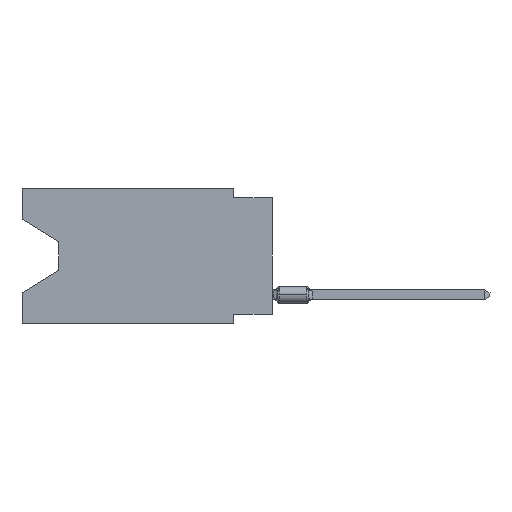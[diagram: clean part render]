
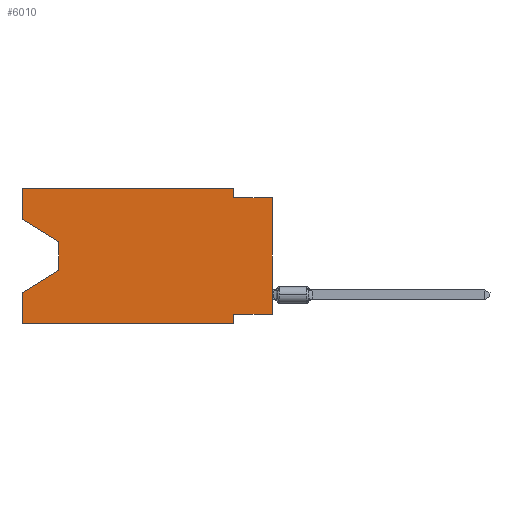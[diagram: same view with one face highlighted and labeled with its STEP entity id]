
A CAD part, left-side view. The second image highlights one B-rep face of the part: STEP entity #6010.
In plain terms, the highlighted planar face has unit normal (-1, 0, 0).
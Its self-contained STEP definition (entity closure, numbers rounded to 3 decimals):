
#204 = VERTEX_POINT ( 'NONE', #6367 ) ;
#647 = DIRECTION ( 'NONE',  ( 0., 1., 0. ) ) ;
#783 = CARTESIAN_POINT ( 'NONE',  ( 0., 0., 0. ) ) ;
#834 = LINE ( 'NONE', #11885, #6127 ) ;
#992 = VECTOR ( 'NONE', #4723, 1000. ) ;
#1112 = ORIENTED_EDGE ( 'NONE', *, *, #3923, .T. ) ;
#1198 = DIRECTION ( 'NONE',  ( 0., 0.855, -0.519 ) ) ;
#1315 = LINE ( 'NONE', #16510, #1983 ) ;
#1483 = CARTESIAN_POINT ( 'NONE',  ( 0., 16.383, -8.89 ) ) ;
#1664 = VECTOR ( 'NONE', #13502, 1000. ) ;
#1983 = VECTOR ( 'NONE', #8372, 1000. ) ;
#2185 = ORIENTED_EDGE ( 'NONE', *, *, #11172, .F. ) ;
#2428 = EDGE_CURVE ( 'NONE', #12531, #3201, #16859, .T. ) ;
#2451 = LINE ( 'NONE', #14931, #11621 ) ;
#2608 = ORIENTED_EDGE ( 'NONE', *, *, #7534, .F. ) ;
#3176 = VERTEX_POINT ( 'NONE', #9819 ) ;
#3201 = VERTEX_POINT ( 'NONE', #9553 ) ;
#3488 = EDGE_CURVE ( 'NONE', #3720, #14097, #834, .T. ) ;
#3533 = ORIENTED_EDGE ( 'NONE', *, *, #11182, .F. ) ;
#3636 = DIRECTION ( 'NONE',  ( 0., 0., 1. ) ) ;
#3705 = CARTESIAN_POINT ( 'NONE',  ( 0., 2.54, -8.89 ) ) ;
#3720 = VERTEX_POINT ( 'NONE', #14129 ) ;
#3766 = FACE_OUTER_BOUND ( 'NONE', #9793, .T. ) ;
#3818 = CARTESIAN_POINT ( 'NONE',  ( 0., 16.383, 0. ) ) ;
#3923 = EDGE_CURVE ( 'NONE', #12180, #12531, #2451, .T. ) ;
#4723 = DIRECTION ( 'NONE',  ( 0., 0., -1. ) ) ;
#4765 = DIRECTION ( 'NONE',  ( 0., 0., 1. ) ) ;
#4813 = VERTEX_POINT ( 'NONE', #16566 ) ;
#5173 = CARTESIAN_POINT ( 'NONE',  ( 0., 16.383, 0. ) ) ;
#5475 = DIRECTION ( 'NONE',  ( 1., 0., 0. ) ) ;
#5490 = CARTESIAN_POINT ( 'NONE',  ( 0., 2.54, 0. ) ) ;
#6010 = ADVANCED_FACE ( 'NONE', ( #3766 ), #17866, .F. ) ;
#6127 = VECTOR ( 'NONE', #647, 1000. ) ;
#6319 = LINE ( 'NONE', #783, #9073 ) ;
#6367 = CARTESIAN_POINT ( 'NONE',  ( 0., 16.383, -6.852 ) ) ;
#6377 = VERTEX_POINT ( 'NONE', #9716 ) ;
#6419 = LINE ( 'NONE', #13300, #14679 ) ;
#6822 = ORIENTED_EDGE ( 'NONE', *, *, #3488, .F. ) ;
#6824 = CARTESIAN_POINT ( 'NONE',  ( 0., 13.97, -5.385 ) ) ;
#6936 = DIRECTION ( 'NONE',  ( 0., 0., -1. ) ) ;
#7210 = CARTESIAN_POINT ( 'NONE',  ( 0., 2.54, -8.255 ) ) ;
#7383 = VERTEX_POINT ( 'NONE', #14224 ) ;
#7534 = EDGE_CURVE ( 'NONE', #12180, #4813, #7885, .T. ) ;
#7779 = DIRECTION ( 'NONE',  ( 0., 0., -1. ) ) ;
#7885 = LINE ( 'NONE', #5173, #16621 ) ;
#8364 = EDGE_CURVE ( 'NONE', #3201, #204, #9628, .T. ) ;
#8372 = DIRECTION ( 'NONE',  ( 0., 0., 1. ) ) ;
#8445 = AXIS2_PLACEMENT_3D ( 'NONE', #16250, #5475, #17686 ) ;
#8815 = CARTESIAN_POINT ( 'NONE',  ( 0., 13.97, -3.505 ) ) ;
#8919 = VECTOR ( 'NONE', #1198, 1000. ) ;
#9073 = VECTOR ( 'NONE', #4765, 1000. ) ;
#9150 = CARTESIAN_POINT ( 'NONE',  ( 0., 0., -0.635 ) ) ;
#9553 = CARTESIAN_POINT ( 'NONE',  ( 0., 13.97, -5.385 ) ) ;
#9628 = LINE ( 'NONE', #6824, #8919 ) ;
#9716 = CARTESIAN_POINT ( 'NONE',  ( 0., 2.54, -0.635 ) ) ;
#9793 = EDGE_LOOP ( 'NONE', ( #1112, #13552, #10392, #10011, #17423, #3533, #6822, #10310, #2185, #11666, #12014, #2608 ) ) ;
#9819 = CARTESIAN_POINT ( 'NONE',  ( 0., 2.54, 0. ) ) ;
#10011 = ORIENTED_EDGE ( 'NONE', *, *, #14334, .F. ) ;
#10019 = VERTEX_POINT ( 'NONE', #9150 ) ;
#10310 = ORIENTED_EDGE ( 'NONE', *, *, #15839, .T. ) ;
#10392 = ORIENTED_EDGE ( 'NONE', *, *, #8364, .T. ) ;
#10852 = VECTOR ( 'NONE', #6936, 1000. ) ;
#10859 = DIRECTION ( 'NONE',  ( 0., -1., 0. ) ) ;
#11172 = EDGE_CURVE ( 'NONE', #6377, #10019, #6419, .T. ) ;
#11182 = EDGE_CURVE ( 'NONE', #14097, #13721, #16277, .T. ) ;
#11621 = VECTOR ( 'NONE', #13398, 1000. ) ;
#11666 = ORIENTED_EDGE ( 'NONE', *, *, #16131, .F. ) ;
#11885 = CARTESIAN_POINT ( 'NONE',  ( 0., 0., -8.255 ) ) ;
#12014 = ORIENTED_EDGE ( 'NONE', *, *, #12551, .F. ) ;
#12160 = CARTESIAN_POINT ( 'NONE',  ( 0., 2.54, -8.89 ) ) ;
#12180 = VERTEX_POINT ( 'NONE', #16938 ) ;
#12291 = LINE ( 'NONE', #5490, #10852 ) ;
#12531 = VERTEX_POINT ( 'NONE', #16300 ) ;
#12551 = EDGE_CURVE ( 'NONE', #4813, #3176, #15033, .T. ) ;
#13300 = CARTESIAN_POINT ( 'NONE',  ( 0., 0., -0.635 ) ) ;
#13398 = DIRECTION ( 'NONE',  ( 0., -0.855, -0.519 ) ) ;
#13502 = DIRECTION ( 'NONE',  ( 0., -1., 0. ) ) ;
#13552 = ORIENTED_EDGE ( 'NONE', *, *, #2428, .T. ) ;
#13721 = VERTEX_POINT ( 'NONE', #12160 ) ;
#14097 = VERTEX_POINT ( 'NONE', #7210 ) ;
#14129 = CARTESIAN_POINT ( 'NONE',  ( 0., 0., -8.255 ) ) ;
#14224 = CARTESIAN_POINT ( 'NONE',  ( 0., 16.383, -8.89 ) ) ;
#14334 = EDGE_CURVE ( 'NONE', #7383, #204, #1315, .T. ) ;
#14411 = EDGE_CURVE ( 'NONE', #7383, #13721, #15157, .T. ) ;
#14679 = VECTOR ( 'NONE', #10859, 1000. ) ;
#14900 = DIRECTION ( 'NONE',  ( 0., -1., 0. ) ) ;
#14931 = CARTESIAN_POINT ( 'NONE',  ( 0., 16.383, -2.038 ) ) ;
#15033 = LINE ( 'NONE', #3818, #1664 ) ;
#15157 = LINE ( 'NONE', #1483, #16146 ) ;
#15839 = EDGE_CURVE ( 'NONE', #3720, #10019, #6319, .T. ) ;
#16131 = EDGE_CURVE ( 'NONE', #3176, #6377, #12291, .T. ) ;
#16146 = VECTOR ( 'NONE', #14900, 1000. ) ;
#16250 = CARTESIAN_POINT ( 'NONE',  ( 0., 16.383, 0. ) ) ;
#16277 = LINE ( 'NONE', #3705, #17565 ) ;
#16300 = CARTESIAN_POINT ( 'NONE',  ( 0., 13.97, -3.505 ) ) ;
#16510 = CARTESIAN_POINT ( 'NONE',  ( 0., 16.383, 0. ) ) ;
#16566 = CARTESIAN_POINT ( 'NONE',  ( 0., 16.383, 0. ) ) ;
#16621 = VECTOR ( 'NONE', #3636, 1000. ) ;
#16859 = LINE ( 'NONE', #8815, #992 ) ;
#16938 = CARTESIAN_POINT ( 'NONE',  ( 0., 16.383, -2.038 ) ) ;
#17423 = ORIENTED_EDGE ( 'NONE', *, *, #14411, .T. ) ;
#17565 = VECTOR ( 'NONE', #7779, 1000. ) ;
#17686 = DIRECTION ( 'NONE',  ( 0., 0., -1. ) ) ;
#17866 = PLANE ( 'NONE',  #8445 ) ;
